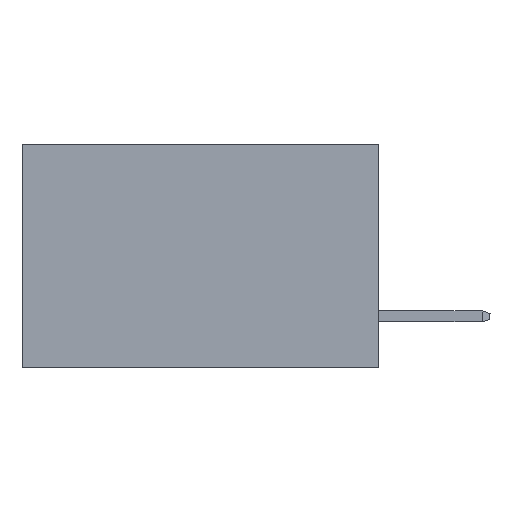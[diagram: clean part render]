
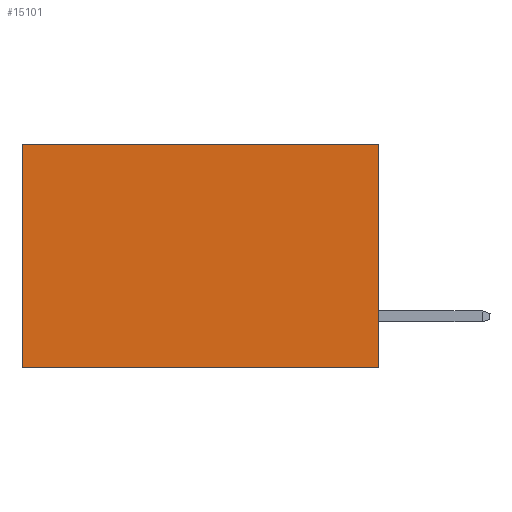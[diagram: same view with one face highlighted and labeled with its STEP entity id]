
A CAD part, left-side view. The second image highlights one B-rep face of the part: STEP entity #15101.
In plain terms, the highlighted planar face has unit normal (-1, 0, 0).
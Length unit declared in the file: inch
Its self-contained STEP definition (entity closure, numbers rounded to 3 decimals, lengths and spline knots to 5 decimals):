
#296 = ORIENTED_EDGE ( 'NONE', *, *, #4135, .T. ) ;
#409 = VERTEX_POINT ( 'NONE', #11737 ) ;
#992 = DIRECTION ( 'NONE',  ( 0., 0., -1. ) ) ;
#1388 = CARTESIAN_POINT ( 'NONE',  ( 0.277, 0.59, -0.37 ) ) ;
#1586 = CARTESIAN_POINT ( 'NONE',  ( 0.277, 0., -0.37 ) ) ;
#1872 = FACE_OUTER_BOUND ( 'NONE', #8219, .T. ) ;
#2485 = VECTOR ( 'NONE', #15418, 39.37008 ) ;
#2723 = AXIS2_PLACEMENT_3D ( 'NONE', #1586, #17410, #8870 ) ;
#3091 = VERTEX_POINT ( 'NONE', #16617 ) ;
#3391 = CARTESIAN_POINT ( 'NONE',  ( 0.277, 0.59, 0. ) ) ;
#3896 = ORIENTED_EDGE ( 'NONE', *, *, #6004, .F. ) ;
#4135 = EDGE_CURVE ( 'NONE', #12792, #14405, #15935, .T. ) ;
#4592 = ORIENTED_EDGE ( 'NONE', *, *, #8333, .T. ) ;
#6004 = EDGE_CURVE ( 'NONE', #409, #14405, #13224, .T. ) ;
#7421 = PLANE ( 'NONE',  #2723 ) ;
#8219 = EDGE_LOOP ( 'NONE', ( #296, #3896, #15369, #4592 ) ) ;
#8333 = EDGE_CURVE ( 'NONE', #3091, #12792, #10199, .T. ) ;
#8870 = DIRECTION ( 'NONE',  ( 0., 0., -1. ) ) ;
#9358 = VECTOR ( 'NONE', #13214, 39.37008 ) ;
#9966 = CARTESIAN_POINT ( 'NONE',  ( 0.277, 0., -0.37 ) ) ;
#10199 = LINE ( 'NONE', #15533, #2485 ) ;
#10676 = EDGE_CURVE ( 'NONE', #3091, #409, #11319, .T. ) ;
#11319 = LINE ( 'NONE', #9966, #17959 ) ;
#11426 = DIRECTION ( 'NONE',  ( 0., 0., -1. ) ) ;
#11737 = CARTESIAN_POINT ( 'NONE',  ( 0.277, 0., -0.37 ) ) ;
#12624 = VECTOR ( 'NONE', #992, 39.37008 ) ;
#12792 = VERTEX_POINT ( 'NONE', #3391 ) ;
#13214 = DIRECTION ( 'NONE',  ( 0., 1., 0. ) ) ;
#13224 = LINE ( 'NONE', #13745, #9358 ) ;
#13745 = CARTESIAN_POINT ( 'NONE',  ( 0.277, 0., -0.37 ) ) ;
#14405 = VERTEX_POINT ( 'NONE', #1388 ) ;
#15101 = ADVANCED_FACE ( 'NONE', ( #1872 ), #7421, .F. ) ;
#15369 = ORIENTED_EDGE ( 'NONE', *, *, #10676, .F. ) ;
#15418 = DIRECTION ( 'NONE',  ( 0., 1., 0. ) ) ;
#15533 = CARTESIAN_POINT ( 'NONE',  ( 0.277, 0., 0. ) ) ;
#15613 = CARTESIAN_POINT ( 'NONE',  ( 0.277, 0.59, -0.37 ) ) ;
#15935 = LINE ( 'NONE', #15613, #12624 ) ;
#16617 = CARTESIAN_POINT ( 'NONE',  ( 0.277, 0., 0. ) ) ;
#17410 = DIRECTION ( 'NONE',  ( 1., 0., 0. ) ) ;
#17959 = VECTOR ( 'NONE', #11426, 39.37008 ) ;
